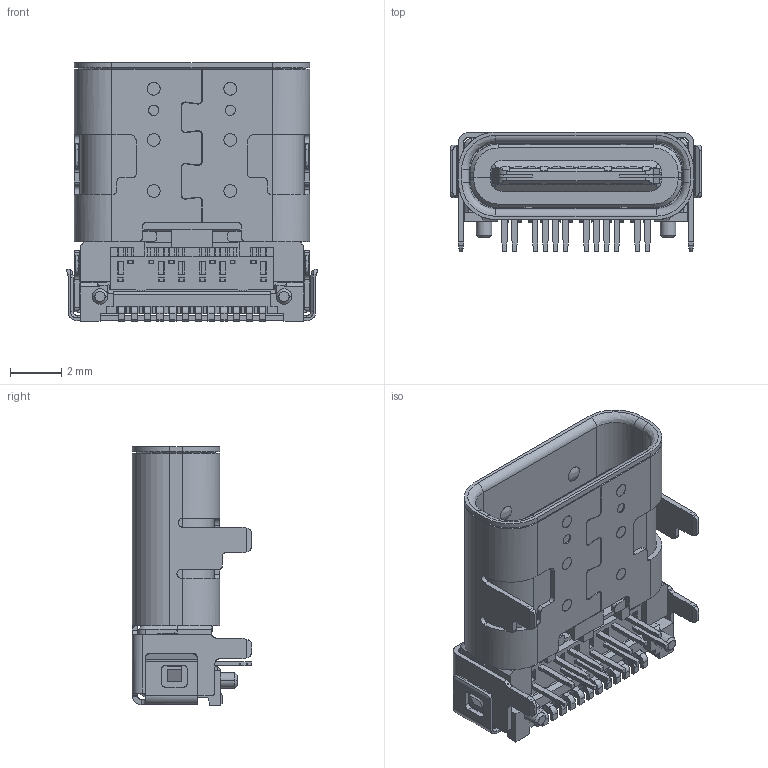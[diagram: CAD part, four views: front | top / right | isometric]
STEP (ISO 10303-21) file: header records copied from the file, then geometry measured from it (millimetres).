
FILE_DESCRIPTION (( 'STEP AP214' ), '1' );
FILE_NAME ('698C124-504-211.STEP', '2021-01-15T17:57:46', ( '' ), ( '' ), 'SwSTEP 2.0', 'SolidWorks 2020', '' );
FILE_SCHEMA (( 'AUTOMOTIVE_DESIGN' ));
Length unit declared in the file: millimetre
Products named in the file (5): Contacts 698C124-504-211; Insulator2 698C124-504-211; Shell 698C124-504-211; Insulator1 698C124-504-211; 698C124-504-211
Assembly tree (4 placements, depth 2):
  698C124-504-211
    Insulator2 698C124-504-211
    Insulator1 698C124-504-211
    Shell 698C124-504-211
    Contacts 698C124-504-211
Bounding box: 9.83 x 4.68 x 10.12 mm (x, y, z)
Volume: 167.3 mm3; surface area: 1503.9 mm2
Topology: 27 solids, 39 shells, 3274 faces, 10015 edges, 6624 vertices
Faces by surface type: plane 2522, cylinder 639, cone 74, bspline 38, torus 1
Entity records: 117386 total; most frequent: CARTESIAN_POINT 31401, ORIENTED_EDGE 20016, DIRECTION 13985, EDGE_CURVE 10008, LINE 7181, VECTOR 7181, VERTEX_POINT 6624, EDGE_LOOP 3440
